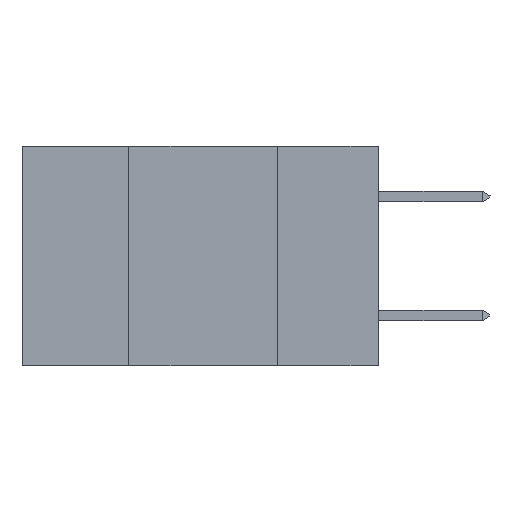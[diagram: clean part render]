
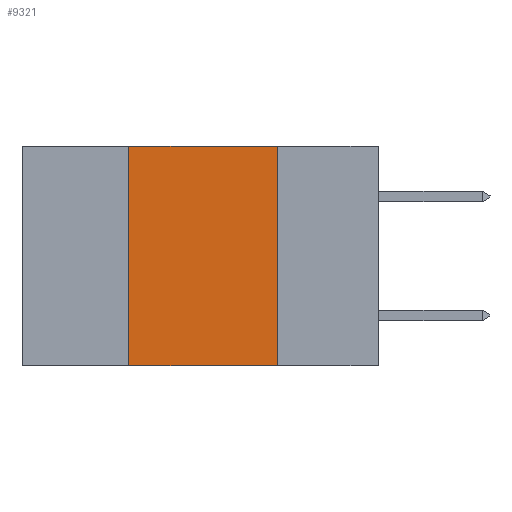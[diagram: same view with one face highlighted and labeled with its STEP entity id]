
A CAD part, left-side view. The second image highlights one B-rep face of the part: STEP entity #9321.
In plain terms, the highlighted planar face has unit normal (-1, 0, 0).
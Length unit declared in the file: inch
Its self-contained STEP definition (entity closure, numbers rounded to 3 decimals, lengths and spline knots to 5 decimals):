
#116 = LINE ( 'NONE', #6390, #11662 ) ;
#492 = LINE ( 'NONE', #15671, #10028 ) ;
#647 = VERTEX_POINT ( 'NONE', #2242 ) ;
#740 = EDGE_CURVE ( 'NONE', #647, #10849, #492, .T. ) ;
#2235 = CARTESIAN_POINT ( 'NONE',  ( 0., 0.17, 0. ) ) ;
#2242 = CARTESIAN_POINT ( 'NONE',  ( 0., 0.42, -0.37 ) ) ;
#2418 = CARTESIAN_POINT ( 'NONE',  ( 0., 0.6, -0.37 ) ) ;
#3809 = PLANE ( 'NONE',  #5022 ) ;
#5022 = AXIS2_PLACEMENT_3D ( 'NONE', #6392, #11550, #12879 ) ;
#5066 = LINE ( 'NONE', #7655, #12578 ) ;
#6310 = DIRECTION ( 'NONE',  ( 0., 0., -1. ) ) ;
#6390 = CARTESIAN_POINT ( 'NONE',  ( 0., 0.6, 0. ) ) ;
#6392 = CARTESIAN_POINT ( 'NONE',  ( 0., 0.6, 0. ) ) ;
#6505 = DIRECTION ( 'NONE',  ( 0., -1., 0. ) ) ;
#6938 = EDGE_LOOP ( 'NONE', ( #8244, #7005, #15978, #10252 ) ) ;
#7005 = ORIENTED_EDGE ( 'NONE', *, *, #9812, .F. ) ;
#7476 = VERTEX_POINT ( 'NONE', #12107 ) ;
#7655 = CARTESIAN_POINT ( 'NONE',  ( 0., 0.17, -0.37 ) ) ;
#8244 = ORIENTED_EDGE ( 'NONE', *, *, #15844, .F. ) ;
#8419 = EDGE_CURVE ( 'NONE', #647, #7476, #12840, .T. ) ;
#9153 = DIRECTION ( 'NONE',  ( 0., 0., 1. ) ) ;
#9321 = ADVANCED_FACE ( 'NONE', ( #15237 ), #3809, .F. ) ;
#9812 = EDGE_CURVE ( 'NONE', #10849, #10361, #116, .T. ) ;
#10028 = VECTOR ( 'NONE', #9153, 39.37008 ) ;
#10252 = ORIENTED_EDGE ( 'NONE', *, *, #8419, .T. ) ;
#10361 = VERTEX_POINT ( 'NONE', #2235 ) ;
#10849 = VERTEX_POINT ( 'NONE', #14688 ) ;
#11550 = DIRECTION ( 'NONE',  ( 1., 0., 0. ) ) ;
#11662 = VECTOR ( 'NONE', #14213, 39.37008 ) ;
#12107 = CARTESIAN_POINT ( 'NONE',  ( 0., 0.17, -0.37 ) ) ;
#12578 = VECTOR ( 'NONE', #6310, 39.37008 ) ;
#12840 = LINE ( 'NONE', #2418, #14569 ) ;
#12879 = DIRECTION ( 'NONE',  ( 0., 0., -1. ) ) ;
#14213 = DIRECTION ( 'NONE',  ( 0., -1., 0. ) ) ;
#14569 = VECTOR ( 'NONE', #6505, 39.37008 ) ;
#14688 = CARTESIAN_POINT ( 'NONE',  ( 0., 0.42, 0. ) ) ;
#15237 = FACE_OUTER_BOUND ( 'NONE', #6938, .T. ) ;
#15671 = CARTESIAN_POINT ( 'NONE',  ( 0., 0.42, -0.37 ) ) ;
#15844 = EDGE_CURVE ( 'NONE', #10361, #7476, #5066, .T. ) ;
#15978 = ORIENTED_EDGE ( 'NONE', *, *, #740, .F. ) ;
